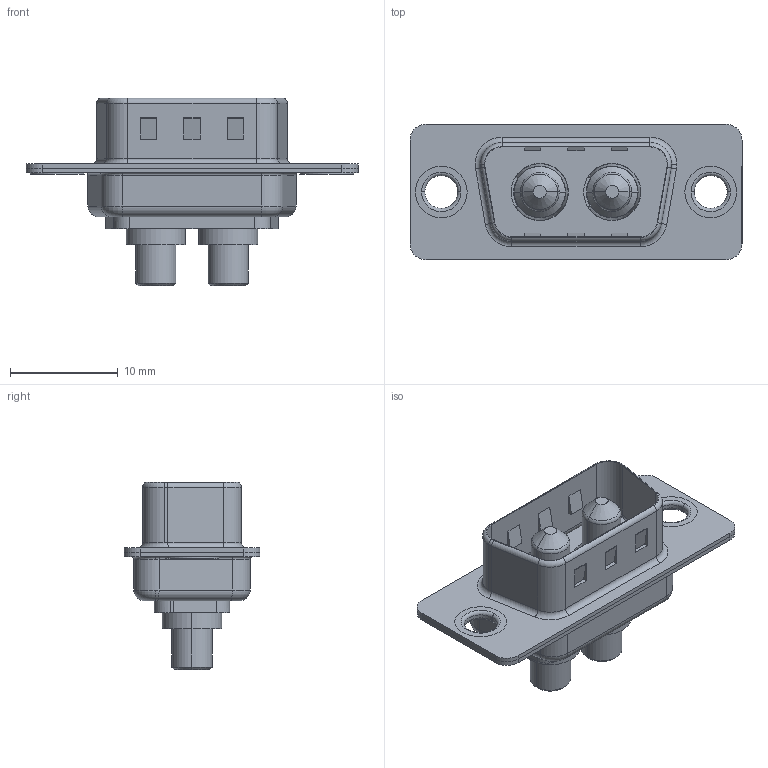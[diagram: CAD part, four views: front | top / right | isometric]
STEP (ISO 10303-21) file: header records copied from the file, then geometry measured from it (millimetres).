
FILE_DESCRIPTION (( 'STEP AP203' ), '1' );
FILE_NAME ('627-2W2-224-4T1.STEP', '2019-05-23T19:56:13', ( '' ), ( '' ), 'SwSTEP 2.0', 'SolidWorks 2016', '' );
FILE_SCHEMA (( 'CONFIG_CONTROL_DESIGN' ));
Length unit declared in the file: millimetre
Products named in the file (6): 627Combo Shell Rear_09 Contacts; 627Combo Shell Front_09 Contacts; 627Combo Thru Hole Rivet; Power Pin_40A S; 627-2W2-224-4T1; 627Combo Housing_2W2
Assembly tree (7 placements, depth 2):
  627-2W2-224-4T1
    627Combo Housing_2W2
    627Combo Shell Rear_09 Contacts
    627Combo Shell Front_09 Contacts
    627Combo Thru Hole Rivet  x2
    Power Pin_40A S  x2
Bounding box: 30.8 x 12.6 x 17.4 mm (x, y, z)
Volume: 1410.9 mm3; surface area: 3468 mm2
Topology: 9 solids, 9 shells, 358 faces, 845 edges, 522 vertices
Faces by surface type: cylinder 151, plane 127, torus 62, cone 14, bspline 4
Entity records: 9652 total; most frequent: DIRECTION 1668, CARTESIAN_POINT 1606, ORIENTED_EDGE 1460, EDGE_CURVE 730, AXIS2_PLACEMENT_3D 646, VERTEX_POINT 454, LINE 376, VECTOR 376
